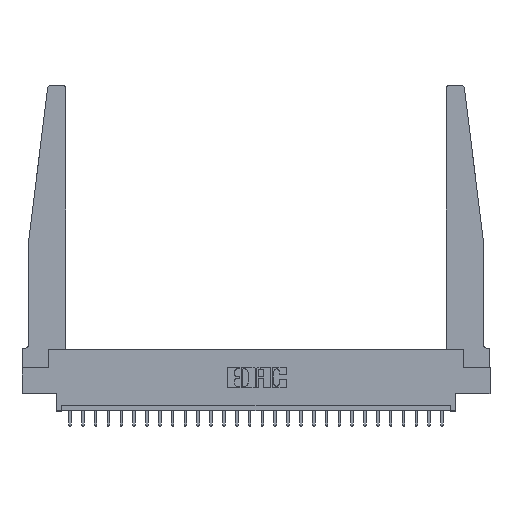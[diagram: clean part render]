
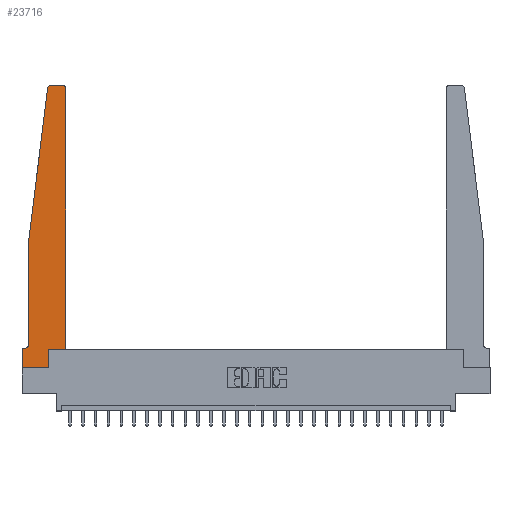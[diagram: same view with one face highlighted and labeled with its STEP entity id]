
A CAD part, top view. The second image highlights one B-rep face of the part: STEP entity #23716.
In plain terms, the highlighted planar face has unit normal (0, 0, 1).
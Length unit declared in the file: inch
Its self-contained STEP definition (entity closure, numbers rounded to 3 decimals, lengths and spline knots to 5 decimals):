
#6 = CARTESIAN_POINT ( 'NONE',  ( 0.015, 0.2375, 0.37 ) ) ;
#394 = VERTEX_POINT ( 'NONE', #1045 ) ;
#961 = EDGE_CURVE ( 'NONE', #22650, #14708, #18026, .T. ) ;
#966 = VERTEX_POINT ( 'NONE', #6018 ) ;
#1045 = CARTESIAN_POINT ( 'NONE',  ( 0.2605, 0.18, 0.37 ) ) ;
#1444 = CARTESIAN_POINT ( 'NONE',  ( 0.2605, 0., 0.37 ) ) ;
#1621 = EDGE_CURVE ( 'NONE', #20353, #14866, #5927, .T. ) ;
#1672 = VECTOR ( 'NONE', #12388, 39.37008 ) ;
#1963 = EDGE_CURVE ( 'NONE', #14708, #3156, #13501, .T. ) ;
#2014 = CARTESIAN_POINT ( 'NONE',  ( 0., 0.1875, 0.37 ) ) ;
#2054 = DIRECTION ( 'NONE',  ( -1., 0., 0. ) ) ;
#2075 = CARTESIAN_POINT ( 'NONE',  ( 0., 0.1875, 0.37 ) ) ;
#2270 = CARTESIAN_POINT ( 'NONE',  ( 0., 0., 0.37 ) ) ;
#2354 = CARTESIAN_POINT ( 'NONE',  ( 0.425, 0.18, 0.37 ) ) ;
#2381 = CARTESIAN_POINT ( 'NONE',  ( 0.065, 1.25, 0.37 ) ) ;
#2560 = EDGE_CURVE ( 'NONE', #22019, #4525, #9053, .T. ) ;
#2903 = CIRCLE ( 'NONE', #22299, 0.03 ) ;
#3156 = VERTEX_POINT ( 'NONE', #9534 ) ;
#3732 = VECTOR ( 'NONE', #14105, 39.37008 ) ;
#4337 = EDGE_CURVE ( 'NONE', #11611, #22019, #12767, .T. ) ;
#4413 = EDGE_CURVE ( 'NONE', #394, #966, #10702, .T. ) ;
#4525 = VERTEX_POINT ( 'NONE', #1444 ) ;
#4603 = CARTESIAN_POINT ( 'NONE',  ( 0.2605, 0.18, 0.37 ) ) ;
#5035 = CARTESIAN_POINT ( 'NONE',  ( 0., 0., 0.37 ) ) ;
#5064 = CARTESIAN_POINT ( 'NONE',  ( 0., 0., 0.37 ) ) ;
#5634 = CIRCLE ( 'NONE', #22998, 0.05 ) ;
#5823 = DIRECTION ( 'NONE',  ( -1., 0., 0. ) ) ;
#5927 = LINE ( 'NONE', #19771, #14498 ) ;
#6018 = CARTESIAN_POINT ( 'NONE',  ( 0.425, 0.18, 0.37 ) ) ;
#6087 = AXIS2_PLACEMENT_3D ( 'NONE', #24484, #14586, #18625 ) ;
#6245 = LINE ( 'NONE', #2354, #3732 ) ;
#6298 = EDGE_CURVE ( 'NONE', #13068, #20353, #2903, .T. ) ;
#6756 = ORIENTED_EDGE ( 'NONE', *, *, #961, .T. ) ;
#6771 = ORIENTED_EDGE ( 'NONE', *, *, #1963, .T. ) ;
#7103 = VECTOR ( 'NONE', #21411, 39.37008 ) ;
#7173 = ORIENTED_EDGE ( 'NONE', *, *, #15676, .T. ) ;
#7399 = EDGE_CURVE ( 'NONE', #966, #13068, #6245, .T. ) ;
#7752 = LINE ( 'NONE', #23569, #14269 ) ;
#8124 = DIRECTION ( 'NONE',  ( -1., 0., 0. ) ) ;
#9053 = LINE ( 'NONE', #5064, #11989 ) ;
#9289 = CARTESIAN_POINT ( 'NONE',  ( 0.27653, 2.75, 0.37 ) ) ;
#9534 = CARTESIAN_POINT ( 'NONE',  ( 0.065, 0.2375, 0.37 ) ) ;
#10696 = VECTOR ( 'NONE', #18609, 39.37008 ) ;
#10702 = LINE ( 'NONE', #14841, #10696 ) ;
#11123 = EDGE_CURVE ( 'NONE', #14866, #22650, #13898, .T. ) ;
#11611 = VERTEX_POINT ( 'NONE', #2014 ) ;
#11986 = DIRECTION ( 'NONE',  ( 1., 0., 0. ) ) ;
#11989 = VECTOR ( 'NONE', #24752, 39.37008 ) ;
#12335 = DIRECTION ( 'NONE',  ( 0., 1., 0. ) ) ;
#12387 = ORIENTED_EDGE ( 'NONE', *, *, #22606, .T. ) ;
#12388 = DIRECTION ( 'NONE',  ( 0., -1., 0. ) ) ;
#12767 = LINE ( 'NONE', #5035, #1672 ) ;
#13068 = VERTEX_POINT ( 'NONE', #23146 ) ;
#13501 = LINE ( 'NONE', #19227, #7103 ) ;
#13527 = CARTESIAN_POINT ( 'NONE',  ( 0.395, 2.75, 0.37 ) ) ;
#13555 = PLANE ( 'NONE',  #18880 ) ;
#13898 = CIRCLE ( 'NONE', #6087, 0.03 ) ;
#13936 = DIRECTION ( 'NONE',  ( 0., 0., 1. ) ) ;
#14105 = DIRECTION ( 'NONE',  ( 0., 1., 0. ) ) ;
#14269 = VECTOR ( 'NONE', #5823, 39.37008 ) ;
#14465 = DIRECTION ( 'NONE',  ( 0., 0., 1. ) ) ;
#14498 = VECTOR ( 'NONE', #2054, 39.37008 ) ;
#14586 = DIRECTION ( 'NONE',  ( 0., 0., 1. ) ) ;
#14708 = VERTEX_POINT ( 'NONE', #2381 ) ;
#14841 = CARTESIAN_POINT ( 'NONE',  ( 0.425, 0.18, 0.37 ) ) ;
#14866 = VERTEX_POINT ( 'NONE', #9289 ) ;
#15676 = EDGE_CURVE ( 'NONE', #4525, #394, #16211, .T. ) ;
#16211 = LINE ( 'NONE', #4603, #25083 ) ;
#16787 = ORIENTED_EDGE ( 'NONE', *, *, #4337, .T. ) ;
#17786 = DIRECTION ( 'NONE',  ( -0.122, -0.992, 0. ) ) ;
#17949 = DIRECTION ( 'NONE',  ( 0., 0., -1. ) ) ;
#18026 = LINE ( 'NONE', #21788, #24038 ) ;
#18154 = ORIENTED_EDGE ( 'NONE', *, *, #6298, .T. ) ;
#18414 = ORIENTED_EDGE ( 'NONE', *, *, #1621, .T. ) ;
#18609 = DIRECTION ( 'NONE',  ( 1., 0., 0. ) ) ;
#18625 = DIRECTION ( 'NONE',  ( 1., 0., 0. ) ) ;
#18634 = VERTEX_POINT ( 'NONE', #19278 ) ;
#18880 = AXIS2_PLACEMENT_3D ( 'NONE', #2075, #13936, #11986 ) ;
#19227 = CARTESIAN_POINT ( 'NONE',  ( 0.065, 1.25, 0.37 ) ) ;
#19278 = CARTESIAN_POINT ( 'NONE',  ( 0.015, 0.1875, 0.37 ) ) ;
#19771 = CARTESIAN_POINT ( 'NONE',  ( 0.25, 2.75, 0.37 ) ) ;
#19873 = ORIENTED_EDGE ( 'NONE', *, *, #11123, .T. ) ;
#19979 = ORIENTED_EDGE ( 'NONE', *, *, #2560, .T. ) ;
#20353 = VERTEX_POINT ( 'NONE', #13527 ) ;
#20622 = CARTESIAN_POINT ( 'NONE',  ( 0.24675, 2.72367, 0.37 ) ) ;
#21079 = ORIENTED_EDGE ( 'NONE', *, *, #7399, .T. ) ;
#21411 = DIRECTION ( 'NONE',  ( 0., -1., 0. ) ) ;
#21788 = CARTESIAN_POINT ( 'NONE',  ( 0.065, 1.25, 0.37 ) ) ;
#22019 = VERTEX_POINT ( 'NONE', #2270 ) ;
#22299 = AXIS2_PLACEMENT_3D ( 'NONE', #22388, #14465, #24737 ) ;
#22309 = ORIENTED_EDGE ( 'NONE', *, *, #4413, .T. ) ;
#22388 = CARTESIAN_POINT ( 'NONE',  ( 0.395, 2.72, 0.37 ) ) ;
#22606 = EDGE_CURVE ( 'NONE', #18634, #11611, #7752, .T. ) ;
#22609 = EDGE_CURVE ( 'NONE', #3156, #18634, #5634, .T. ) ;
#22650 = VERTEX_POINT ( 'NONE', #20622 ) ;
#22998 = AXIS2_PLACEMENT_3D ( 'NONE', #6, #17949, #8124 ) ;
#23146 = CARTESIAN_POINT ( 'NONE',  ( 0.425, 2.72, 0.37 ) ) ;
#23569 = CARTESIAN_POINT ( 'NONE',  ( 0.065, 0.1875, 0.37 ) ) ;
#23716 = ADVANCED_FACE ( 'NONE', ( #25504 ), #13555, .T. ) ;
#23965 = ORIENTED_EDGE ( 'NONE', *, *, #22609, .T. ) ;
#24038 = VECTOR ( 'NONE', #17786, 39.37008 ) ;
#24283 = EDGE_LOOP ( 'NONE', ( #18414, #19873, #6756, #6771, #23965, #12387, #16787, #19979, #7173, #22309, #21079, #18154 ) ) ;
#24484 = CARTESIAN_POINT ( 'NONE',  ( 0.27653, 2.72, 0.37 ) ) ;
#24737 = DIRECTION ( 'NONE',  ( 1., 0., 0. ) ) ;
#24752 = DIRECTION ( 'NONE',  ( 1., 0., 0. ) ) ;
#25083 = VECTOR ( 'NONE', #12335, 39.37008 ) ;
#25504 = FACE_OUTER_BOUND ( 'NONE', #24283, .T. ) ;
